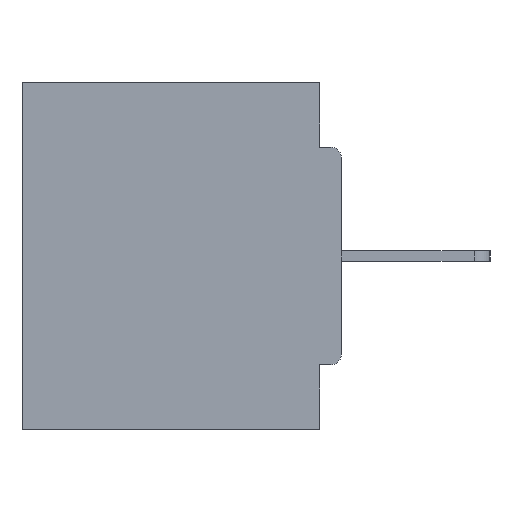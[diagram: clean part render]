
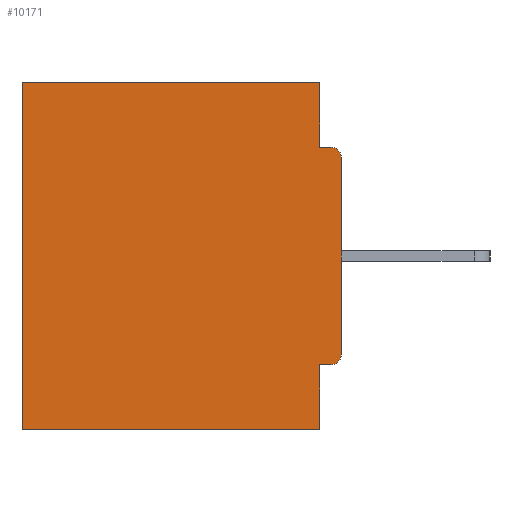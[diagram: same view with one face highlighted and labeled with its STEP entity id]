
A CAD part, left-side view. The second image highlights one B-rep face of the part: STEP entity #10171.
In plain terms, the highlighted planar face has unit normal (-1, 0, 0).
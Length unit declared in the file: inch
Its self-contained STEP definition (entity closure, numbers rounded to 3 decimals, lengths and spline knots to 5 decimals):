
#383 = CARTESIAN_POINT ( 'NONE',  ( 0.298, 0.46, 0. ) ) ;
#691 = DIRECTION ( 'NONE',  ( 0., 1., 0. ) ) ;
#792 = ORIENTED_EDGE ( 'NONE', *, *, #21354, .T. ) ;
#1463 = CARTESIAN_POINT ( 'NONE',  ( 0.298, 0., -0.1085 ) ) ;
#1886 = CARTESIAN_POINT ( 'NONE',  ( 0.298, 0., -0.0935 ) ) ;
#2349 = CARTESIAN_POINT ( 'NONE',  ( 0.298, 0., -0.3915 ) ) ;
#2518 = EDGE_CURVE ( 'NONE', #19315, #3074, #16746, .T. ) ;
#3042 = ORIENTED_EDGE ( 'NONE', *, *, #8423, .F. ) ;
#3074 = VERTEX_POINT ( 'NONE', #13467 ) ;
#3745 = EDGE_CURVE ( 'NONE', #9884, #10637, #11394, .T. ) ;
#4469 = AXIS2_PLACEMENT_3D ( 'NONE', #32638, #28645, #28812 ) ;
#4863 = AXIS2_PLACEMENT_3D ( 'NONE', #27256, #11884, #29903 ) ;
#5555 = ORIENTED_EDGE ( 'NONE', *, *, #12136, .T. ) ;
#6167 = CARTESIAN_POINT ( 'NONE',  ( 0.298, 0.46, -0.5 ) ) ;
#6264 = ORIENTED_EDGE ( 'NONE', *, *, #20736, .F. ) ;
#6648 = LINE ( 'NONE', #31438, #26380 ) ;
#6787 = CARTESIAN_POINT ( 'NONE',  ( 0.298, 0.031, -0.4065 ) ) ;
#6924 = VERTEX_POINT ( 'NONE', #11258 ) ;
#7676 = DIRECTION ( 'NONE',  ( 0., 0., -1. ) ) ;
#8097 = DIRECTION ( 'NONE',  ( 0., 0., -1. ) ) ;
#8423 = EDGE_CURVE ( 'NONE', #15320, #23080, #22143, .T. ) ;
#8478 = EDGE_CURVE ( 'NONE', #19315, #9720, #27440, .T. ) ;
#9720 = VERTEX_POINT ( 'NONE', #2349 ) ;
#9884 = VERTEX_POINT ( 'NONE', #10689 ) ;
#10171 = ADVANCED_FACE ( 'NONE', ( #21665 ), #22127, .F. ) ;
#10637 = VERTEX_POINT ( 'NONE', #6167 ) ;
#10689 = CARTESIAN_POINT ( 'NONE',  ( 0.298, 0.031, -0.5 ) ) ;
#10899 = ORIENTED_EDGE ( 'NONE', *, *, #27052, .F. ) ;
#11258 = CARTESIAN_POINT ( 'NONE',  ( 0.298, 0.015, -0.4065 ) ) ;
#11365 = VERTEX_POINT ( 'NONE', #20059 ) ;
#11394 = LINE ( 'NONE', #21052, #17490 ) ;
#11884 = DIRECTION ( 'NONE',  ( 1., 0., 0. ) ) ;
#11996 = DIRECTION ( 'NONE',  ( -1., 0., 0. ) ) ;
#12136 = EDGE_CURVE ( 'NONE', #15320, #11365, #29585, .T. ) ;
#12166 = ORIENTED_EDGE ( 'NONE', *, *, #16612, .F. ) ;
#13199 = DIRECTION ( 'NONE',  ( 0., 1., 0. ) ) ;
#13467 = CARTESIAN_POINT ( 'NONE',  ( 0.298, 0.015, -0.0935 ) ) ;
#14149 = CARTESIAN_POINT ( 'NONE',  ( 0.298, 0.031, -0.0935 ) ) ;
#14918 = VECTOR ( 'NONE', #25059, 39.37008 ) ;
#15320 = VERTEX_POINT ( 'NONE', #27352 ) ;
#15703 = CARTESIAN_POINT ( 'NONE',  ( 0.298, 0., 0. ) ) ;
#16612 = EDGE_CURVE ( 'NONE', #25915, #9884, #23097, .T. ) ;
#16746 = CIRCLE ( 'NONE', #4469, 0.015 ) ;
#16823 = ORIENTED_EDGE ( 'NONE', *, *, #3745, .F. ) ;
#17407 = CARTESIAN_POINT ( 'NONE',  ( 0.298, 0., 0. ) ) ;
#17490 = VECTOR ( 'NONE', #19414, 39.37008 ) ;
#17777 = DIRECTION ( 'NONE',  ( 0., 0., -1. ) ) ;
#19315 = VERTEX_POINT ( 'NONE', #1463 ) ;
#19414 = DIRECTION ( 'NONE',  ( 0., 1., 0. ) ) ;
#20059 = CARTESIAN_POINT ( 'NONE',  ( 0.298, 0.46, 0. ) ) ;
#20538 = DIRECTION ( 'NONE',  ( 0., 0., -1. ) ) ;
#20648 = CARTESIAN_POINT ( 'NONE',  ( 0.298, 0.031, -0.5 ) ) ;
#20736 = EDGE_CURVE ( 'NONE', #23080, #3074, #21746, .T. ) ;
#21052 = CARTESIAN_POINT ( 'NONE',  ( 0.298, 0., -0.5 ) ) ;
#21354 = EDGE_CURVE ( 'NONE', #6924, #9720, #22914, .T. ) ;
#21471 = VECTOR ( 'NONE', #7676, 39.37008 ) ;
#21665 = FACE_OUTER_BOUND ( 'NONE', #25453, .T. ) ;
#21746 = LINE ( 'NONE', #1886, #14918 ) ;
#22127 = PLANE ( 'NONE',  #4863 ) ;
#22143 = LINE ( 'NONE', #20648, #29021 ) ;
#22440 = AXIS2_PLACEMENT_3D ( 'NONE', #27479, #11996, #30012 ) ;
#22710 = VECTOR ( 'NONE', #13199, 39.37008 ) ;
#22914 = CIRCLE ( 'NONE', #22440, 0.015 ) ;
#23042 = CARTESIAN_POINT ( 'NONE',  ( 0.298, 0.031, -0.5 ) ) ;
#23080 = VERTEX_POINT ( 'NONE', #14149 ) ;
#23097 = LINE ( 'NONE', #23042, #21471 ) ;
#25059 = DIRECTION ( 'NONE',  ( 0., -1., 0. ) ) ;
#25453 = EDGE_LOOP ( 'NONE', ( #29573, #6264, #3042, #5555, #31843, #16823, #12166, #10899, #792, #27510 ) ) ;
#25851 = VECTOR ( 'NONE', #17777, 39.37008 ) ;
#25915 = VERTEX_POINT ( 'NONE', #6787 ) ;
#26380 = VECTOR ( 'NONE', #691, 39.37008 ) ;
#27052 = EDGE_CURVE ( 'NONE', #6924, #25915, #6648, .T. ) ;
#27256 = CARTESIAN_POINT ( 'NONE',  ( 0.298, 0., 0. ) ) ;
#27352 = CARTESIAN_POINT ( 'NONE',  ( 0.298, 0.031, 0. ) ) ;
#27440 = LINE ( 'NONE', #17407, #25851 ) ;
#27479 = CARTESIAN_POINT ( 'NONE',  ( 0.298, 0.015, -0.3915 ) ) ;
#27510 = ORIENTED_EDGE ( 'NONE', *, *, #8478, .F. ) ;
#28209 = LINE ( 'NONE', #383, #32530 ) ;
#28645 = DIRECTION ( 'NONE',  ( -1., 0., 0. ) ) ;
#28812 = DIRECTION ( 'NONE',  ( 0., 0., -1. ) ) ;
#29021 = VECTOR ( 'NONE', #20538, 39.37008 ) ;
#29412 = EDGE_CURVE ( 'NONE', #11365, #10637, #28209, .T. ) ;
#29573 = ORIENTED_EDGE ( 'NONE', *, *, #2518, .T. ) ;
#29585 = LINE ( 'NONE', #15703, #22710 ) ;
#29903 = DIRECTION ( 'NONE',  ( 0., 0., -1. ) ) ;
#30012 = DIRECTION ( 'NONE',  ( 0., 0., -1. ) ) ;
#31438 = CARTESIAN_POINT ( 'NONE',  ( 0.298, 0., -0.4065 ) ) ;
#31843 = ORIENTED_EDGE ( 'NONE', *, *, #29412, .T. ) ;
#32530 = VECTOR ( 'NONE', #8097, 39.37008 ) ;
#32638 = CARTESIAN_POINT ( 'NONE',  ( 0.298, 0.015, -0.1085 ) ) ;
